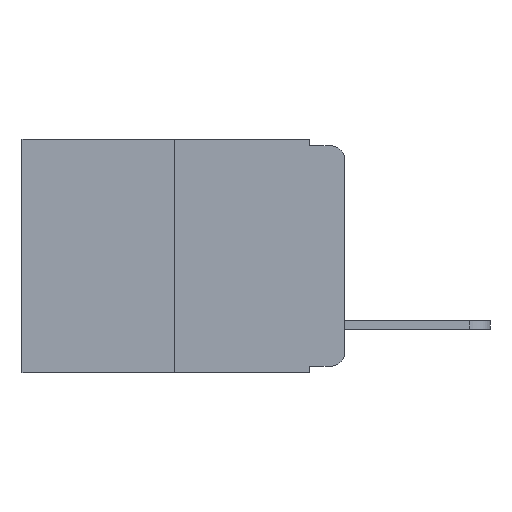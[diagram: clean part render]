
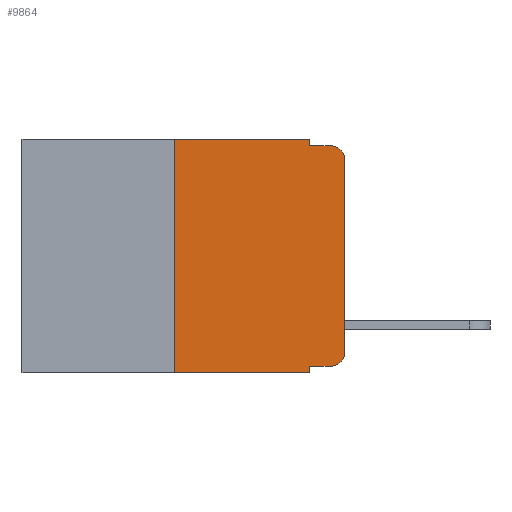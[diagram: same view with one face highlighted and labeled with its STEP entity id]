
A CAD part, left-side view. The second image highlights one B-rep face of the part: STEP entity #9864.
In plain terms, the highlighted planar face has unit normal (-1, 0, 0).
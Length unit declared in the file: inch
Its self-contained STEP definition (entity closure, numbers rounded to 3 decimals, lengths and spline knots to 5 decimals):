
#1003 = DIRECTION ( 'NONE',  ( 0., 0., 1. ) ) ;
#1215 = VERTEX_POINT ( 'NONE', #9081 ) ;
#1356 = CARTESIAN_POINT ( 'NONE',  ( 0., 0.473, -0.343 ) ) ;
#1765 = EDGE_CURVE ( 'NONE', #16208, #12858, #3978, .T. ) ;
#2063 = EDGE_CURVE ( 'NONE', #12775, #14195, #11120, .T. ) ;
#2233 = CARTESIAN_POINT ( 'NONE',  ( 0., 0.25, 0. ) ) ;
#2465 = DIRECTION ( 'NONE',  ( 0., 0., -1. ) ) ;
#3134 = EDGE_CURVE ( 'NONE', #19035, #12775, #5091, .T. ) ;
#3405 = AXIS2_PLACEMENT_3D ( 'NONE', #11862, #13520, #17909 ) ;
#3618 = DIRECTION ( 'NONE',  ( 0., 0., -1. ) ) ;
#3978 = LINE ( 'NONE', #1356, #13272 ) ;
#5091 = LINE ( 'NONE', #19093, #16275 ) ;
#5179 = EDGE_CURVE ( 'NONE', #1215, #12858, #10272, .T. ) ;
#5537 = ORIENTED_EDGE ( 'NONE', *, *, #5679, .F. ) ;
#5679 = EDGE_CURVE ( 'NONE', #14195, #18737, #6677, .T. ) ;
#5689 = VECTOR ( 'NONE', #17291, 39.37008 ) ;
#5932 = CARTESIAN_POINT ( 'NONE',  ( 0., 0.051, -0.343 ) ) ;
#6187 = EDGE_CURVE ( 'NONE', #12771, #10823, #11650, .T. ) ;
#6211 = EDGE_CURVE ( 'NONE', #16208, #19035, #18730, .T. ) ;
#6285 = CARTESIAN_POINT ( 'NONE',  ( 0., 0.051, -0.01 ) ) ;
#6677 = LINE ( 'NONE', #14355, #5689 ) ;
#6760 = VECTOR ( 'NONE', #16948, 39.37008 ) ;
#6958 = ORIENTED_EDGE ( 'NONE', *, *, #5179, .F. ) ;
#7092 = CARTESIAN_POINT ( 'NONE',  ( 0., 0.25, 0. ) ) ;
#7702 = VERTEX_POINT ( 'NONE', #9227 ) ;
#8174 = AXIS2_PLACEMENT_3D ( 'NONE', #13341, #17676, #10343 ) ;
#8195 = CARTESIAN_POINT ( 'NONE',  ( 0., 0.051, 0. ) ) ;
#8508 = CIRCLE ( 'NONE', #8789, 0.02 ) ;
#8646 = CARTESIAN_POINT ( 'NONE',  ( 0., 0., 0. ) ) ;
#8723 = ORIENTED_EDGE ( 'NONE', *, *, #19272, .T. ) ;
#8789 = AXIS2_PLACEMENT_3D ( 'NONE', #10177, #14585, #2465 ) ;
#9081 = CARTESIAN_POINT ( 'NONE',  ( 0., 0.051, -0.333 ) ) ;
#9227 = CARTESIAN_POINT ( 'NONE',  ( 0., 0.02, -0.333 ) ) ;
#9864 = ADVANCED_FACE ( 'NONE', ( #17017 ), #10324, .F. ) ;
#10142 = DIRECTION ( 'NONE',  ( 0., 0., 1. ) ) ;
#10177 = CARTESIAN_POINT ( 'NONE',  ( 0., 0.02, -0.03 ) ) ;
#10272 = LINE ( 'NONE', #16337, #13128 ) ;
#10324 = PLANE ( 'NONE',  #3405 ) ;
#10343 = DIRECTION ( 'NONE',  ( 0., 0., -1. ) ) ;
#10610 = EDGE_CURVE ( 'NONE', #10823, #18737, #8508, .T. ) ;
#10823 = VERTEX_POINT ( 'NONE', #15114 ) ;
#10884 = CARTESIAN_POINT ( 'NONE',  ( 0., 0.25, -0.343 ) ) ;
#10970 = CARTESIAN_POINT ( 'NONE',  ( 0., 0.051, 0. ) ) ;
#11024 = ORIENTED_EDGE ( 'NONE', *, *, #2063, .F. ) ;
#11120 = LINE ( 'NONE', #8195, #12091 ) ;
#11176 = VECTOR ( 'NONE', #1003, 39.37008 ) ;
#11645 = DIRECTION ( 'NONE',  ( 0., -1., 0. ) ) ;
#11650 = LINE ( 'NONE', #8646, #12834 ) ;
#11715 = DIRECTION ( 'NONE',  ( 0., 0., -1. ) ) ;
#11862 = CARTESIAN_POINT ( 'NONE',  ( 0., 0.473, 0. ) ) ;
#12091 = VECTOR ( 'NONE', #3618, 39.37008 ) ;
#12771 = VERTEX_POINT ( 'NONE', #15704 ) ;
#12775 = VERTEX_POINT ( 'NONE', #10970 ) ;
#12834 = VECTOR ( 'NONE', #10142, 39.37008 ) ;
#12858 = VERTEX_POINT ( 'NONE', #5932 ) ;
#13128 = VECTOR ( 'NONE', #11715, 39.37008 ) ;
#13218 = ORIENTED_EDGE ( 'NONE', *, *, #6187, .T. ) ;
#13251 = ORIENTED_EDGE ( 'NONE', *, *, #16339, .T. ) ;
#13272 = VECTOR ( 'NONE', #16564, 39.37008 ) ;
#13341 = CARTESIAN_POINT ( 'NONE',  ( 0., 0.02, -0.313 ) ) ;
#13503 = ORIENTED_EDGE ( 'NONE', *, *, #6211, .F. ) ;
#13520 = DIRECTION ( 'NONE',  ( 1., 0., 0. ) ) ;
#14195 = VERTEX_POINT ( 'NONE', #6285 ) ;
#14215 = CARTESIAN_POINT ( 'NONE',  ( 0., 0.051, -0.333 ) ) ;
#14355 = CARTESIAN_POINT ( 'NONE',  ( 0., 0.051, -0.01 ) ) ;
#14384 = LINE ( 'NONE', #14215, #6760 ) ;
#14492 = EDGE_LOOP ( 'NONE', ( #13218, #14731, #5537, #11024, #19480, #13503, #16884, #6958, #13251, #8723 ) ) ;
#14585 = DIRECTION ( 'NONE',  ( -1., 0., 0. ) ) ;
#14731 = ORIENTED_EDGE ( 'NONE', *, *, #10610, .T. ) ;
#15114 = CARTESIAN_POINT ( 'NONE',  ( 0., 0., -0.03 ) ) ;
#15704 = CARTESIAN_POINT ( 'NONE',  ( 0., 0., -0.313 ) ) ;
#16208 = VERTEX_POINT ( 'NONE', #10884 ) ;
#16275 = VECTOR ( 'NONE', #11645, 39.37008 ) ;
#16337 = CARTESIAN_POINT ( 'NONE',  ( 0., 0.051, 0. ) ) ;
#16339 = EDGE_CURVE ( 'NONE', #1215, #7702, #14384, .T. ) ;
#16564 = DIRECTION ( 'NONE',  ( 0., -1., 0. ) ) ;
#16884 = ORIENTED_EDGE ( 'NONE', *, *, #1765, .T. ) ;
#16948 = DIRECTION ( 'NONE',  ( 0., -1., 0. ) ) ;
#17017 = FACE_OUTER_BOUND ( 'NONE', #14492, .T. ) ;
#17291 = DIRECTION ( 'NONE',  ( 0., -1., 0. ) ) ;
#17555 = CIRCLE ( 'NONE', #8174, 0.02 ) ;
#17676 = DIRECTION ( 'NONE',  ( -1., 0., 0. ) ) ;
#17909 = DIRECTION ( 'NONE',  ( 0., 0., -1. ) ) ;
#18257 = CARTESIAN_POINT ( 'NONE',  ( 0., 0.02, -0.01 ) ) ;
#18730 = LINE ( 'NONE', #7092, #11176 ) ;
#18737 = VERTEX_POINT ( 'NONE', #18257 ) ;
#19035 = VERTEX_POINT ( 'NONE', #2233 ) ;
#19093 = CARTESIAN_POINT ( 'NONE',  ( 0., 0.473, 0. ) ) ;
#19272 = EDGE_CURVE ( 'NONE', #7702, #12771, #17555, .T. ) ;
#19480 = ORIENTED_EDGE ( 'NONE', *, *, #3134, .F. ) ;
